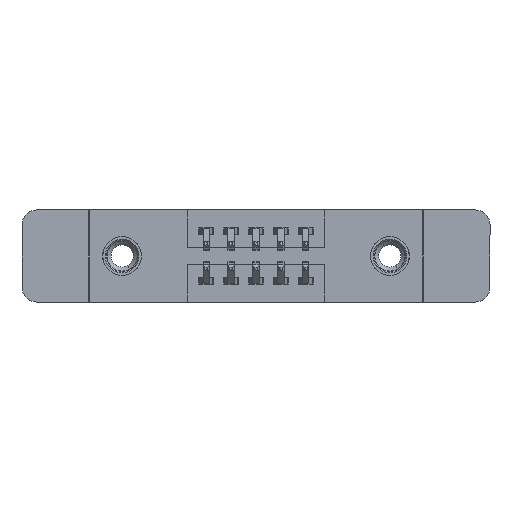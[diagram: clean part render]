
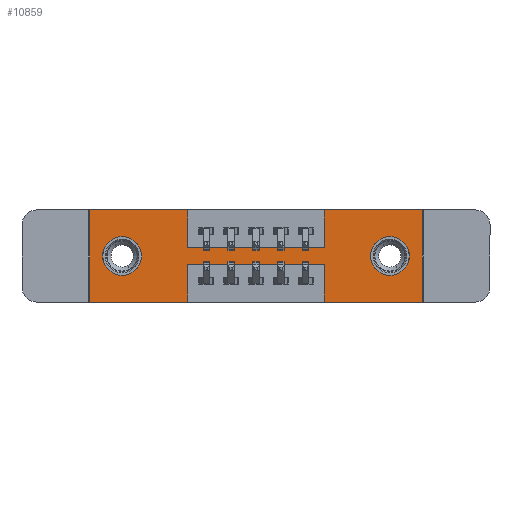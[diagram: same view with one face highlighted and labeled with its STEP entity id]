
A CAD part, front view. The second image highlights one B-rep face of the part: STEP entity #10859.
In plain terms, the highlighted planar face has unit normal (0, -1, 0).
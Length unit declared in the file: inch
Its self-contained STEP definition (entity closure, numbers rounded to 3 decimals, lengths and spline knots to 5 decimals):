
#59 = LINE ( 'NONE', #4558, #6291 ) ;
#348 = EDGE_LOOP ( 'NONE', ( #12077, #7898 ) ) ;
#365 = DIRECTION ( 'NONE',  ( 0., 0., 1. ) ) ;
#430 = VECTOR ( 'NONE', #7086, 39.37008 ) ;
#442 = LINE ( 'NONE', #5065, #11883 ) ;
#477 = DIRECTION ( 'NONE',  ( 0., 0., -1. ) ) ;
#588 = CARTESIAN_POINT ( 'NONE',  ( 0., 0., 0. ) ) ;
#738 = VERTEX_POINT ( 'NONE', #6524 ) ;
#899 = ORIENTED_EDGE ( 'NONE', *, *, #8607, .F. ) ;
#1128 = VERTEX_POINT ( 'NONE', #12090 ) ;
#1199 = EDGE_CURVE ( 'NONE', #1128, #8879, #3622, .T. ) ;
#1463 = ORIENTED_EDGE ( 'NONE', *, *, #1807, .F. ) ;
#1473 = CARTESIAN_POINT ( 'NONE',  ( 0.3925, 0., -0.15 ) ) ;
#1689 = VERTEX_POINT ( 'NONE', #13280 ) ;
#1807 = EDGE_CURVE ( 'NONE', #11756, #12246, #12950, .T. ) ;
#1906 = LINE ( 'NONE', #588, #2948 ) ;
#1996 = LINE ( 'NONE', #1473, #430 ) ;
#2020 = CARTESIAN_POINT ( 'NONE',  ( 1.335, 0., 0. ) ) ;
#2118 = ORIENTED_EDGE ( 'NONE', *, *, #8099, .F. ) ;
#2342 = EDGE_CURVE ( 'NONE', #8879, #1128, #6190, .T. ) ;
#2349 = CARTESIAN_POINT ( 'NONE',  ( 0., 0., 0. ) ) ;
#2546 = DIRECTION ( 'NONE',  ( 0., 0., 1. ) ) ;
#2561 = EDGE_LOOP ( 'NONE', ( #10906, #7529 ) ) ;
#2636 = CARTESIAN_POINT ( 'NONE',  ( 0.13, 0., -0.185 ) ) ;
#2673 = CIRCLE ( 'NONE', #3609, 0.078 ) ;
#2930 = CARTESIAN_POINT ( 'NONE',  ( 0.3925, 0., -0.22 ) ) ;
#2948 = VECTOR ( 'NONE', #3991, 39.37008 ) ;
#2952 = DIRECTION ( 'NONE',  ( 0., 0., -1. ) ) ;
#2955 = ORIENTED_EDGE ( 'NONE', *, *, #5064, .F. ) ;
#3045 = VERTEX_POINT ( 'NONE', #7852 ) ;
#3231 = EDGE_CURVE ( 'NONE', #3045, #1689, #442, .T. ) ;
#3456 = VECTOR ( 'NONE', #7549, 39.37008 ) ;
#3476 = CARTESIAN_POINT ( 'NONE',  ( 0., 0., -0.37 ) ) ;
#3499 = EDGE_CURVE ( 'NONE', #9264, #12478, #1996, .T. ) ;
#3592 = CARTESIAN_POINT ( 'NONE',  ( 0.13, 0., -0.185 ) ) ;
#3609 = AXIS2_PLACEMENT_3D ( 'NONE', #3592, #4709, #10186 ) ;
#3622 = CIRCLE ( 'NONE', #11827, 0.078 ) ;
#3672 = DIRECTION ( 'NONE',  ( 0., 0., 1. ) ) ;
#3684 = LINE ( 'NONE', #10945, #8022 ) ;
#3932 = DIRECTION ( 'NONE',  ( 0., 0., 1. ) ) ;
#3991 = DIRECTION ( 'NONE',  ( 1., 0., 0. ) ) ;
#4064 = EDGE_CURVE ( 'NONE', #4789, #9837, #2673, .T. ) ;
#4274 = VECTOR ( 'NONE', #3932, 39.37008 ) ;
#4558 = CARTESIAN_POINT ( 'NONE',  ( 0.3925, 0., -0.37 ) ) ;
#4688 = DIRECTION ( 'NONE',  ( 0., 1., 0. ) ) ;
#4709 = DIRECTION ( 'NONE',  ( 0., 1., 0. ) ) ;
#4734 = CARTESIAN_POINT ( 'NONE',  ( 1.205, 0., -0.185 ) ) ;
#4789 = VERTEX_POINT ( 'NONE', #12952 ) ;
#4913 = EDGE_CURVE ( 'NONE', #12246, #5525, #3684, .T. ) ;
#5064 = EDGE_CURVE ( 'NONE', #13950, #6504, #59, .T. ) ;
#5065 = CARTESIAN_POINT ( 'NONE',  ( 0., 0., -0.37 ) ) ;
#5217 = DIRECTION ( 'NONE',  ( 0., 0., -1. ) ) ;
#5525 = VERTEX_POINT ( 'NONE', #8414 ) ;
#5837 = FACE_BOUND ( 'NONE', #348, .T. ) ;
#6190 = CIRCLE ( 'NONE', #13222, 0.078 ) ;
#6262 = ORIENTED_EDGE ( 'NONE', *, *, #3499, .F. ) ;
#6291 = VECTOR ( 'NONE', #6736, 39.37008 ) ;
#6504 = VERTEX_POINT ( 'NONE', #6933 ) ;
#6524 = CARTESIAN_POINT ( 'NONE',  ( 0.9425, 0., -0.22 ) ) ;
#6707 = CARTESIAN_POINT ( 'NONE',  ( 1.205, 0., -0.107 ) ) ;
#6736 = DIRECTION ( 'NONE',  ( 0., 0., -1. ) ) ;
#6867 = EDGE_LOOP ( 'NONE', ( #2955, #6941, #7491, #9912, #7386, #899, #9612, #6262, #2118, #10550, #1463, #13106 ) ) ;
#6881 = VECTOR ( 'NONE', #7107, 39.37008 ) ;
#6933 = CARTESIAN_POINT ( 'NONE',  ( 0.3925, 0., -0.37 ) ) ;
#6941 = ORIENTED_EDGE ( 'NONE', *, *, #9859, .F. ) ;
#6962 = CARTESIAN_POINT ( 'NONE',  ( 0.9425, 0., -0.37 ) ) ;
#7086 = DIRECTION ( 'NONE',  ( 1., 0., 0. ) ) ;
#7107 = DIRECTION ( 'NONE',  ( -1., 0., 0. ) ) ;
#7199 = LINE ( 'NONE', #10607, #4274 ) ;
#7386 = ORIENTED_EDGE ( 'NONE', *, *, #9547, .F. ) ;
#7491 = ORIENTED_EDGE ( 'NONE', *, *, #7627, .F. ) ;
#7529 = ORIENTED_EDGE ( 'NONE', *, *, #1199, .T. ) ;
#7549 = DIRECTION ( 'NONE',  ( -1., 0., 0. ) ) ;
#7563 = CIRCLE ( 'NONE', #9427, 0.078 ) ;
#7627 = EDGE_CURVE ( 'NONE', #1689, #738, #9747, .T. ) ;
#7799 = LINE ( 'NONE', #2930, #3456 ) ;
#7852 = CARTESIAN_POINT ( 'NONE',  ( 1.335, 0., -0.37 ) ) ;
#7898 = ORIENTED_EDGE ( 'NONE', *, *, #4064, .T. ) ;
#7974 = CARTESIAN_POINT ( 'NONE',  ( 0.9425, 0., 0. ) ) ;
#8022 = VECTOR ( 'NONE', #12042, 39.37008 ) ;
#8071 = LINE ( 'NONE', #12706, #6881 ) ;
#8099 = EDGE_CURVE ( 'NONE', #5525, #9264, #14032, .T. ) ;
#8152 = CARTESIAN_POINT ( 'NONE',  ( 0.3925, 0., -0.22 ) ) ;
#8290 = VECTOR ( 'NONE', #10354, 39.37008 ) ;
#8414 = CARTESIAN_POINT ( 'NONE',  ( 0.3925, 0., 0. ) ) ;
#8597 = CARTESIAN_POINT ( 'NONE',  ( 0.13, 0., -0.107 ) ) ;
#8607 = EDGE_CURVE ( 'NONE', #11710, #9868, #1906, .T. ) ;
#8772 = AXIS2_PLACEMENT_3D ( 'NONE', #9585, #9481, #2952 ) ;
#8879 = VERTEX_POINT ( 'NONE', #6707 ) ;
#9193 = CARTESIAN_POINT ( 'NONE',  ( 0., 0., 0. ) ) ;
#9204 = VECTOR ( 'NONE', #2546, 39.37008 ) ;
#9264 = VERTEX_POINT ( 'NONE', #9578 ) ;
#9427 = AXIS2_PLACEMENT_3D ( 'NONE', #2636, #13561, #365 ) ;
#9481 = DIRECTION ( 'NONE',  ( 0., -1., 0. ) ) ;
#9547 = EDGE_CURVE ( 'NONE', #9868, #3045, #13317, .T. ) ;
#9578 = CARTESIAN_POINT ( 'NONE',  ( 0.3925, 0., -0.15 ) ) ;
#9585 = CARTESIAN_POINT ( 'NONE',  ( 0., 0., -0.37 ) ) ;
#9612 = ORIENTED_EDGE ( 'NONE', *, *, #12443, .F. ) ;
#9670 = DIRECTION ( 'NONE',  ( -1., 0., 0. ) ) ;
#9731 = VECTOR ( 'NONE', #5217, 39.37008 ) ;
#9747 = LINE ( 'NONE', #6962, #9204 ) ;
#9837 = VERTEX_POINT ( 'NONE', #8597 ) ;
#9859 = EDGE_CURVE ( 'NONE', #738, #13950, #7799, .T. ) ;
#9868 = VERTEX_POINT ( 'NONE', #2020 ) ;
#9912 = ORIENTED_EDGE ( 'NONE', *, *, #3231, .F. ) ;
#10186 = DIRECTION ( 'NONE',  ( 0., 0., 1. ) ) ;
#10354 = DIRECTION ( 'NONE',  ( 0., 0., -1. ) ) ;
#10550 = ORIENTED_EDGE ( 'NONE', *, *, #4913, .F. ) ;
#10607 = CARTESIAN_POINT ( 'NONE',  ( 0.9425, 0., 0. ) ) ;
#10653 = PLANE ( 'NONE',  #8772 ) ;
#10677 = FACE_OUTER_BOUND ( 'NONE', #6867, .T. ) ;
#10859 = ADVANCED_FACE ( 'NONE', ( #11224, #5837, #10677 ), #10653, .T. ) ;
#10906 = ORIENTED_EDGE ( 'NONE', *, *, #2342, .T. ) ;
#10945 = CARTESIAN_POINT ( 'NONE',  ( 0., 0., 0. ) ) ;
#11224 = FACE_BOUND ( 'NONE', #2561, .T. ) ;
#11579 = VECTOR ( 'NONE', #3672, 39.37008 ) ;
#11710 = VERTEX_POINT ( 'NONE', #7974 ) ;
#11756 = VERTEX_POINT ( 'NONE', #3476 ) ;
#11773 = CARTESIAN_POINT ( 'NONE',  ( 1.205, 0., -0.185 ) ) ;
#11827 = AXIS2_PLACEMENT_3D ( 'NONE', #11773, #12873, #477 ) ;
#11883 = VECTOR ( 'NONE', #9670, 39.37008 ) ;
#12042 = DIRECTION ( 'NONE',  ( 1., 0., 0. ) ) ;
#12077 = ORIENTED_EDGE ( 'NONE', *, *, #13968, .T. ) ;
#12090 = CARTESIAN_POINT ( 'NONE',  ( 1.205, 0., -0.263 ) ) ;
#12246 = VERTEX_POINT ( 'NONE', #2349 ) ;
#12419 = DIRECTION ( 'NONE',  ( 0., 0., -1. ) ) ;
#12443 = EDGE_CURVE ( 'NONE', #12478, #11710, #7199, .T. ) ;
#12478 = VERTEX_POINT ( 'NONE', #12812 ) ;
#12514 = CARTESIAN_POINT ( 'NONE',  ( 1.335, 0., 0. ) ) ;
#12706 = CARTESIAN_POINT ( 'NONE',  ( 0., 0., -0.37 ) ) ;
#12812 = CARTESIAN_POINT ( 'NONE',  ( 0.9425, 0., -0.15 ) ) ;
#12873 = DIRECTION ( 'NONE',  ( 0., 1., 0. ) ) ;
#12950 = LINE ( 'NONE', #9193, #11579 ) ;
#12952 = CARTESIAN_POINT ( 'NONE',  ( 0.13, 0., -0.263 ) ) ;
#12991 = CARTESIAN_POINT ( 'NONE',  ( 0.3925, 0., 0. ) ) ;
#13106 = ORIENTED_EDGE ( 'NONE', *, *, #13504, .F. ) ;
#13222 = AXIS2_PLACEMENT_3D ( 'NONE', #4734, #4688, #12419 ) ;
#13280 = CARTESIAN_POINT ( 'NONE',  ( 0.9425, 0., -0.37 ) ) ;
#13317 = LINE ( 'NONE', #12514, #8290 ) ;
#13504 = EDGE_CURVE ( 'NONE', #6504, #11756, #8071, .T. ) ;
#13561 = DIRECTION ( 'NONE',  ( 0., 1., 0. ) ) ;
#13950 = VERTEX_POINT ( 'NONE', #8152 ) ;
#13968 = EDGE_CURVE ( 'NONE', #9837, #4789, #7563, .T. ) ;
#14032 = LINE ( 'NONE', #12991, #9731 ) ;
